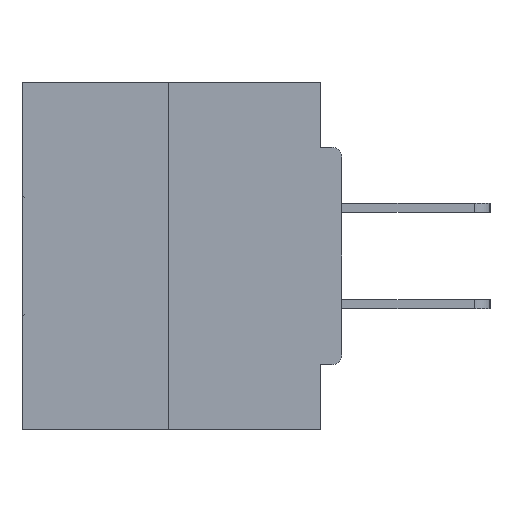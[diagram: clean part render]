
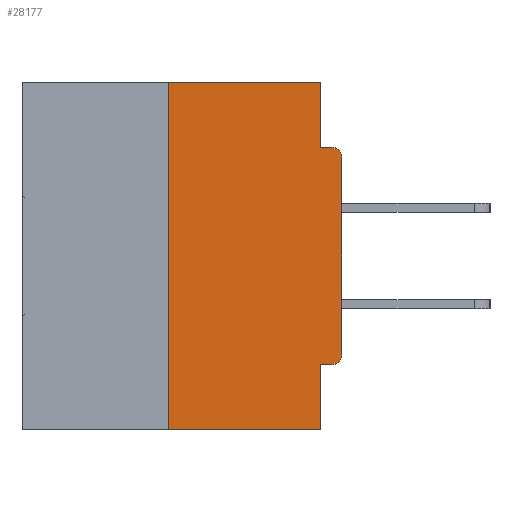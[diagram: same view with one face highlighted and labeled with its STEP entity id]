
A CAD part, left-side view. The second image highlights one B-rep face of the part: STEP entity #28177.
In plain terms, the highlighted planar face has unit normal (-1, 0, 0).
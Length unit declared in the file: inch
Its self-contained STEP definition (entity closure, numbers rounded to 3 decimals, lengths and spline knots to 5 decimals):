
#84 = VERTEX_POINT ( 'NONE', #36717 ) ;
#222 = DIRECTION ( 'NONE',  ( 0., 0., -1. ) ) ;
#1339 = VERTEX_POINT ( 'NONE', #38610 ) ;
#1488 = LINE ( 'NONE', #14119, #37075 ) ;
#2130 = VERTEX_POINT ( 'NONE', #25836 ) ;
#2634 = ORIENTED_EDGE ( 'NONE', *, *, #14212, .F. ) ;
#2723 = CARTESIAN_POINT ( 'NONE',  ( 0., 0.031, -0.5 ) ) ;
#2876 = LINE ( 'NONE', #37089, #21855 ) ;
#3088 = ORIENTED_EDGE ( 'NONE', *, *, #6422, .T. ) ;
#4720 = DIRECTION ( 'NONE',  ( 0., 0., 1. ) ) ;
#5487 = VECTOR ( 'NONE', #12300, 39.37008 ) ;
#5710 = ORIENTED_EDGE ( 'NONE', *, *, #17705, .T. ) ;
#5866 = CIRCLE ( 'NONE', #36961, 0.015 ) ;
#6422 = EDGE_CURVE ( 'NONE', #84, #2130, #26847, .T. ) ;
#7524 = EDGE_CURVE ( 'NONE', #14214, #30559, #32212, .T. ) ;
#8108 = EDGE_LOOP ( 'NONE', ( #30276, #13876, #26235, #40842, #40472, #10597, #3088, #5710, #28453, #2634 ) ) ;
#8289 = DIRECTION ( 'NONE',  ( 0., -1., 0. ) ) ;
#8586 = LINE ( 'NONE', #40723, #5487 ) ;
#10597 = ORIENTED_EDGE ( 'NONE', *, *, #17869, .T. ) ;
#10736 = LINE ( 'NONE', #19849, #39172 ) ;
#11369 = EDGE_CURVE ( 'NONE', #34104, #26944, #1488, .T. ) ;
#12062 = VECTOR ( 'NONE', #25736, 39.37008 ) ;
#12300 = DIRECTION ( 'NONE',  ( 0., 1., 0. ) ) ;
#12463 = DIRECTION ( 'NONE',  ( 1., 0., 0. ) ) ;
#13019 = DIRECTION ( 'NONE',  ( -1., 0., 0. ) ) ;
#13548 = CARTESIAN_POINT ( 'NONE',  ( 0., 0.031, 0. ) ) ;
#13876 = ORIENTED_EDGE ( 'NONE', *, *, #18044, .F. ) ;
#14119 = CARTESIAN_POINT ( 'NONE',  ( 0., 0., -0.0935 ) ) ;
#14212 = EDGE_CURVE ( 'NONE', #30559, #34104, #10736, .T. ) ;
#14214 = VERTEX_POINT ( 'NONE', #26309 ) ;
#16037 = CARTESIAN_POINT ( 'NONE',  ( 0., 0.46, 0. ) ) ;
#16373 = CARTESIAN_POINT ( 'NONE',  ( 0., 0.015, -0.0935 ) ) ;
#16741 = DIRECTION ( 'NONE',  ( 0., 0., -1. ) ) ;
#17705 = EDGE_CURVE ( 'NONE', #2130, #26944, #5866, .T. ) ;
#17869 = EDGE_CURVE ( 'NONE', #21055, #84, #27115, .T. ) ;
#18044 = EDGE_CURVE ( 'NONE', #1339, #14214, #32722, .T. ) ;
#18959 = VECTOR ( 'NONE', #28716, 39.37008 ) ;
#19077 = EDGE_CURVE ( 'NONE', #1339, #28065, #2876, .T. ) ;
#19799 = VECTOR ( 'NONE', #4720, 39.37008 ) ;
#19849 = CARTESIAN_POINT ( 'NONE',  ( 0., 0.031, 0. ) ) ;
#20311 = VECTOR ( 'NONE', #30155, 39.37008 ) ;
#20466 = AXIS2_PLACEMENT_3D ( 'NONE', #28603, #13019, #25073 ) ;
#20481 = CARTESIAN_POINT ( 'NONE',  ( 0., 0.25, 0. ) ) ;
#21055 = VERTEX_POINT ( 'NONE', #26079 ) ;
#21855 = VECTOR ( 'NONE', #8289, 39.37008 ) ;
#25073 = DIRECTION ( 'NONE',  ( 0., 0., -1. ) ) ;
#25736 = DIRECTION ( 'NONE',  ( 0., 0., -1. ) ) ;
#25836 = CARTESIAN_POINT ( 'NONE',  ( 0., 0., -0.1085 ) ) ;
#26079 = CARTESIAN_POINT ( 'NONE',  ( 0., 0.015, -0.4065 ) ) ;
#26235 = ORIENTED_EDGE ( 'NONE', *, *, #19077, .T. ) ;
#26309 = CARTESIAN_POINT ( 'NONE',  ( 0., 0.25, 0. ) ) ;
#26805 = DIRECTION ( 'NONE',  ( 0., -1., 0. ) ) ;
#26847 = LINE ( 'NONE', #33261, #20311 ) ;
#26944 = VERTEX_POINT ( 'NONE', #16373 ) ;
#27115 = CIRCLE ( 'NONE', #20466, 0.015 ) ;
#28065 = VERTEX_POINT ( 'NONE', #2723 ) ;
#28177 = ADVANCED_FACE ( 'NONE', ( #31746 ), #37755, .F. ) ;
#28453 = ORIENTED_EDGE ( 'NONE', *, *, #11369, .F. ) ;
#28603 = CARTESIAN_POINT ( 'NONE',  ( 0., 0.015, -0.3915 ) ) ;
#28716 = DIRECTION ( 'NONE',  ( 0., -1., 0. ) ) ;
#28834 = LINE ( 'NONE', #32127, #12062 ) ;
#30057 = CARTESIAN_POINT ( 'NONE',  ( 0., 0.031, -0.0935 ) ) ;
#30155 = DIRECTION ( 'NONE',  ( 0., 0., 1. ) ) ;
#30276 = ORIENTED_EDGE ( 'NONE', *, *, #7524, .F. ) ;
#30559 = VERTEX_POINT ( 'NONE', #13548 ) ;
#31297 = VERTEX_POINT ( 'NONE', #40383 ) ;
#31746 = FACE_OUTER_BOUND ( 'NONE', #8108, .T. ) ;
#32127 = CARTESIAN_POINT ( 'NONE',  ( 0., 0.031, -0.5 ) ) ;
#32212 = LINE ( 'NONE', #16037, #18959 ) ;
#32722 = LINE ( 'NONE', #20481, #19799 ) ;
#33261 = CARTESIAN_POINT ( 'NONE',  ( 0., 0., 0. ) ) ;
#33581 = AXIS2_PLACEMENT_3D ( 'NONE', #35251, #12463, #222 ) ;
#33978 = CARTESIAN_POINT ( 'NONE',  ( 0., 0.015, -0.1085 ) ) ;
#34104 = VERTEX_POINT ( 'NONE', #30057 ) ;
#34178 = DIRECTION ( 'NONE',  ( -1., 0., 0. ) ) ;
#35251 = CARTESIAN_POINT ( 'NONE',  ( 0., 0.46, 0. ) ) ;
#35338 = EDGE_CURVE ( 'NONE', #31297, #28065, #28834, .T. ) ;
#36717 = CARTESIAN_POINT ( 'NONE',  ( 0., 0., -0.3915 ) ) ;
#36961 = AXIS2_PLACEMENT_3D ( 'NONE', #33978, #34178, #39814 ) ;
#37075 = VECTOR ( 'NONE', #26805, 39.37008 ) ;
#37089 = CARTESIAN_POINT ( 'NONE',  ( 0., 0.46, -0.5 ) ) ;
#37755 = PLANE ( 'NONE',  #33581 ) ;
#38610 = CARTESIAN_POINT ( 'NONE',  ( 0., 0.25, -0.5 ) ) ;
#39172 = VECTOR ( 'NONE', #16741, 39.37008 ) ;
#39814 = DIRECTION ( 'NONE',  ( 0., 0., -1. ) ) ;
#40383 = CARTESIAN_POINT ( 'NONE',  ( 0., 0.031, -0.4065 ) ) ;
#40472 = ORIENTED_EDGE ( 'NONE', *, *, #40543, .F. ) ;
#40543 = EDGE_CURVE ( 'NONE', #21055, #31297, #8586, .T. ) ;
#40723 = CARTESIAN_POINT ( 'NONE',  ( 0., 0., -0.4065 ) ) ;
#40842 = ORIENTED_EDGE ( 'NONE', *, *, #35338, .F. ) ;
